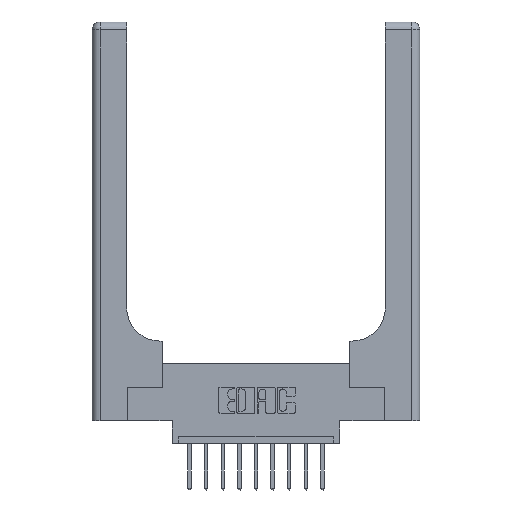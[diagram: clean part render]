
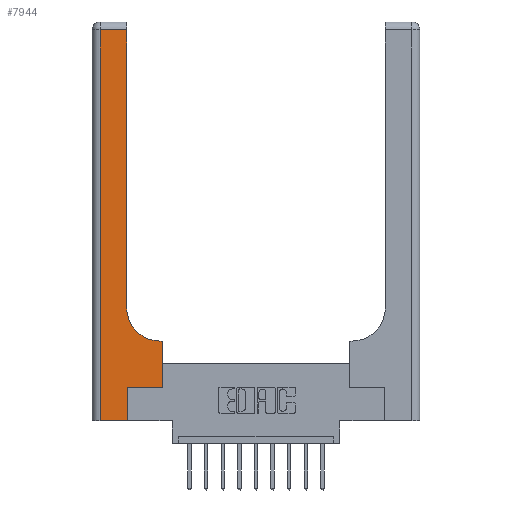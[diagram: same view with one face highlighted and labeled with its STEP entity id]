
A CAD part, top view. The second image highlights one B-rep face of the part: STEP entity #7944.
In plain terms, the highlighted planar face has unit normal (0, 0, 1).
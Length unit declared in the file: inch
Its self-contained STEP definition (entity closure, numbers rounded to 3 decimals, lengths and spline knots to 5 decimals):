
#52 = VERTEX_POINT ( 'NONE', #114 ) ;
#114 = CARTESIAN_POINT ( 'NONE',  ( 0.265, 0.25, 0.37 ) ) ;
#209 = VERTEX_POINT ( 'NONE', #2422 ) ;
#290 = AXIS2_PLACEMENT_3D ( 'NONE', #606, #13674, #2985 ) ;
#309 = CARTESIAN_POINT ( 'NONE',  ( 0.26, 3., 0.37 ) ) ;
#424 = ORIENTED_EDGE ( 'NONE', *, *, #12639, .T. ) ;
#426 = FACE_OUTER_BOUND ( 'NONE', #5874, .T. ) ;
#606 = CARTESIAN_POINT ( 'NONE',  ( 0., 3., 0.37 ) ) ;
#785 = VECTOR ( 'NONE', #6473, 39.37008 ) ;
#1037 = CIRCLE ( 'NONE', #11041, 0.25 ) ;
#1159 = CARTESIAN_POINT ( 'NONE',  ( 0.26, 0.6, 0.37 ) ) ;
#1219 = CARTESIAN_POINT ( 'NONE',  ( 0.26, 0.85, 0.37 ) ) ;
#2116 = VERTEX_POINT ( 'NONE', #6662 ) ;
#2422 = CARTESIAN_POINT ( 'NONE',  ( 0.528, 0.6, 0.37 ) ) ;
#2689 = CARTESIAN_POINT ( 'NONE',  ( 0.06, 2.94, 0.37 ) ) ;
#2761 = CARTESIAN_POINT ( 'NONE',  ( 0.265, 0.25, 0.37 ) ) ;
#2762 = DIRECTION ( 'NONE',  ( 0., 0., -1. ) ) ;
#2985 = DIRECTION ( 'NONE',  ( -1., 0., 0. ) ) ;
#3092 = VECTOR ( 'NONE', #7467, 39.37008 ) ;
#3229 = LINE ( 'NONE', #14064, #15299 ) ;
#3708 = EDGE_CURVE ( 'NONE', #5454, #13645, #14139, .T. ) ;
#3773 = VECTOR ( 'NONE', #14961, 39.37008 ) ;
#3813 = ORIENTED_EDGE ( 'NONE', *, *, #4868, .T. ) ;
#3962 = CARTESIAN_POINT ( 'NONE',  ( 0.51, 0.6, 0.37 ) ) ;
#4394 = LINE ( 'NONE', #7972, #11816 ) ;
#4580 = ORIENTED_EDGE ( 'NONE', *, *, #13907, .T. ) ;
#4657 = ORIENTED_EDGE ( 'NONE', *, *, #6730, .T. ) ;
#4868 = EDGE_CURVE ( 'NONE', #52, #2116, #9877, .T. ) ;
#5033 = CARTESIAN_POINT ( 'NONE',  ( 0.06, 3., 0.37 ) ) ;
#5034 = VECTOR ( 'NONE', #7436, 39.37008 ) ;
#5242 = DIRECTION ( 'NONE',  ( 0., 1., 0. ) ) ;
#5254 = VECTOR ( 'NONE', #5242, 39.37008 ) ;
#5442 = CARTESIAN_POINT ( 'NONE',  ( 0.06, 0., 0.37 ) ) ;
#5454 = VERTEX_POINT ( 'NONE', #1219 ) ;
#5500 = ORIENTED_EDGE ( 'NONE', *, *, #8038, .T. ) ;
#5510 = VERTEX_POINT ( 'NONE', #2689 ) ;
#5874 = EDGE_LOOP ( 'NONE', ( #6899, #5500, #9498, #7241, #424, #3813, #7811, #4580, #4657 ) ) ;
#6473 = DIRECTION ( 'NONE',  ( 1., 0., 0. ) ) ;
#6647 = CARTESIAN_POINT ( 'NONE',  ( 0.26, 2.94, 0.37 ) ) ;
#6662 = CARTESIAN_POINT ( 'NONE',  ( 0.528, 0.25, 0.37 ) ) ;
#6730 = EDGE_CURVE ( 'NONE', #6769, #5454, #1037, .T. ) ;
#6769 = VERTEX_POINT ( 'NONE', #3962 ) ;
#6899 = ORIENTED_EDGE ( 'NONE', *, *, #3708, .T. ) ;
#7188 = LINE ( 'NONE', #5033, #3092 ) ;
#7241 = ORIENTED_EDGE ( 'NONE', *, *, #14194, .T. ) ;
#7436 = DIRECTION ( 'NONE',  ( 1., 0., 0. ) ) ;
#7467 = DIRECTION ( 'NONE',  ( 0., -1., 0. ) ) ;
#7811 = ORIENTED_EDGE ( 'NONE', *, *, #13503, .T. ) ;
#7944 = ADVANCED_FACE ( 'NONE', ( #426 ), #12537, .F. ) ;
#7972 = CARTESIAN_POINT ( 'NONE',  ( 0.265, 0., 0.37 ) ) ;
#8038 = EDGE_CURVE ( 'NONE', #13645, #5510, #13974, .T. ) ;
#8161 = DIRECTION ( 'NONE',  ( 0., 1., 0. ) ) ;
#8582 = VERTEX_POINT ( 'NONE', #15086 ) ;
#9498 = ORIENTED_EDGE ( 'NONE', *, *, #12505, .T. ) ;
#9877 = LINE ( 'NONE', #2761, #5034 ) ;
#9952 = DIRECTION ( 'NONE',  ( 1., 0., 0. ) ) ;
#10115 = CARTESIAN_POINT ( 'NONE',  ( 0.51, 0.85, 0.37 ) ) ;
#10334 = DIRECTION ( 'NONE',  ( 0., 1., 0. ) ) ;
#11041 = AXIS2_PLACEMENT_3D ( 'NONE', #10115, #2762, #9952 ) ;
#11402 = CARTESIAN_POINT ( 'NONE',  ( 0., 2.94, 0.37 ) ) ;
#11775 = VECTOR ( 'NONE', #12961, 39.37008 ) ;
#11816 = VECTOR ( 'NONE', #10334, 39.37008 ) ;
#12505 = EDGE_CURVE ( 'NONE', #5510, #12806, #7188, .T. ) ;
#12537 = PLANE ( 'NONE',  #290 ) ;
#12639 = EDGE_CURVE ( 'NONE', #8582, #52, #4394, .T. ) ;
#12806 = VERTEX_POINT ( 'NONE', #5442 ) ;
#12961 = DIRECTION ( 'NONE',  ( -1., 0., 0. ) ) ;
#13466 = CARTESIAN_POINT ( 'NONE',  ( 0., 0., 0.37 ) ) ;
#13503 = EDGE_CURVE ( 'NONE', #2116, #209, #3229, .T. ) ;
#13645 = VERTEX_POINT ( 'NONE', #6647 ) ;
#13674 = DIRECTION ( 'NONE',  ( 0., 0., -1. ) ) ;
#13907 = EDGE_CURVE ( 'NONE', #209, #6769, #14550, .T. ) ;
#13974 = LINE ( 'NONE', #11402, #3773 ) ;
#14064 = CARTESIAN_POINT ( 'NONE',  ( 0.528, 0.25, 0.37 ) ) ;
#14139 = LINE ( 'NONE', #309, #5254 ) ;
#14194 = EDGE_CURVE ( 'NONE', #12806, #8582, #14530, .T. ) ;
#14530 = LINE ( 'NONE', #13466, #785 ) ;
#14550 = LINE ( 'NONE', #1159, #11775 ) ;
#14961 = DIRECTION ( 'NONE',  ( -1., 0., 0. ) ) ;
#15086 = CARTESIAN_POINT ( 'NONE',  ( 0.265, 0., 0.37 ) ) ;
#15299 = VECTOR ( 'NONE', #8161, 39.37008 ) ;
